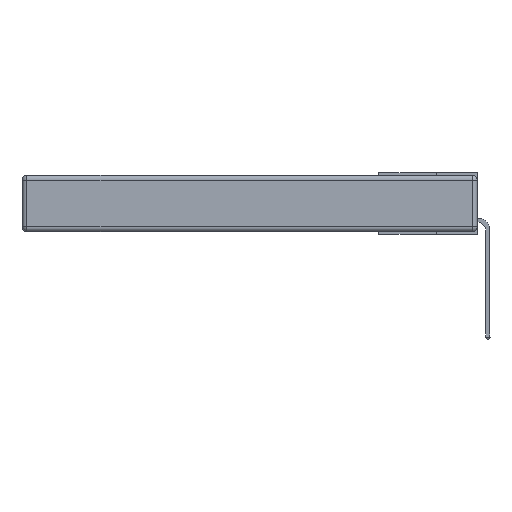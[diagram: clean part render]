
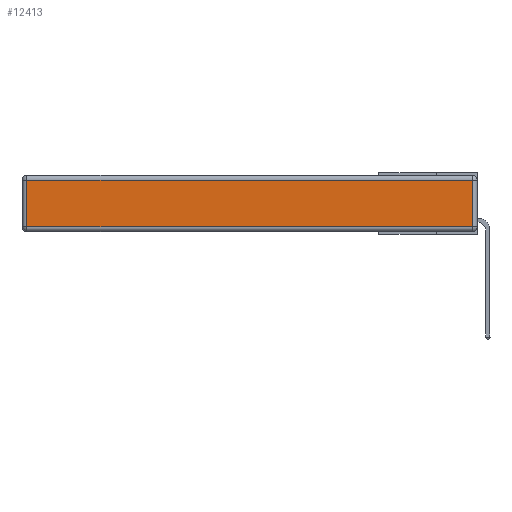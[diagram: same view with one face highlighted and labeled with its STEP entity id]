
A CAD part, left-side view. The second image highlights one B-rep face of the part: STEP entity #12413.
In plain terms, the highlighted planar face has unit normal (-1, 0, 0).
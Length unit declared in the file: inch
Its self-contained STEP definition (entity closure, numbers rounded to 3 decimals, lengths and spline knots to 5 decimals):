
#301 = CARTESIAN_POINT ( 'NONE',  ( 0., 2.75, -0.03 ) ) ;
#462 = LINE ( 'NONE', #27082, #18370 ) ;
#1208 = LINE ( 'NONE', #301, #10140 ) ;
#1718 = DIRECTION ( 'NONE',  ( -1., 0., 0. ) ) ;
#2941 = ORIENTED_EDGE ( 'NONE', *, *, #12968, .T. ) ;
#3369 = CARTESIAN_POINT ( 'NONE',  ( 0., 2.72, -0.03 ) ) ;
#3749 = VECTOR ( 'NONE', #17147, 39.37008 ) ;
#4694 = ORIENTED_EDGE ( 'NONE', *, *, #11218, .T. ) ;
#5098 = VERTEX_POINT ( 'NONE', #3369 ) ;
#5734 = CARTESIAN_POINT ( 'NONE',  ( 0., 0., -0.313 ) ) ;
#6032 = AXIS2_PLACEMENT_3D ( 'NONE', #13320, #1718, #24806 ) ;
#7993 = EDGE_CURVE ( 'NONE', #5098, #28779, #23115, .T. ) ;
#8801 = DIRECTION ( 'NONE',  ( 0., 0., -1. ) ) ;
#9459 = VERTEX_POINT ( 'NONE', #27248 ) ;
#10140 = VECTOR ( 'NONE', #11590, 39.37008 ) ;
#10469 = FACE_OUTER_BOUND ( 'NONE', #27353, .T. ) ;
#11218 = EDGE_CURVE ( 'NONE', #28779, #9459, #20643, .T. ) ;
#11470 = EDGE_CURVE ( 'NONE', #28701, #5098, #1208, .T. ) ;
#11590 = DIRECTION ( 'NONE',  ( 0., 1., 0. ) ) ;
#12413 = ADVANCED_FACE ( 'NONE', ( #10469 ), #15328, .T. ) ;
#12968 = EDGE_CURVE ( 'NONE', #9459, #28701, #462, .T. ) ;
#12983 = CARTESIAN_POINT ( 'NONE',  ( 0., 2.72, -0.313 ) ) ;
#13287 = DIRECTION ( 'NONE',  ( 0., 0., 1. ) ) ;
#13320 = CARTESIAN_POINT ( 'NONE',  ( 0., 0., -0.343 ) ) ;
#13616 = CARTESIAN_POINT ( 'NONE',  ( 0., 2.72, -0.343 ) ) ;
#15328 = PLANE ( 'NONE',  #6032 ) ;
#17147 = DIRECTION ( 'NONE',  ( 0., -1., 0. ) ) ;
#18370 = VECTOR ( 'NONE', #13287, 39.37008 ) ;
#20643 = LINE ( 'NONE', #5734, #3749 ) ;
#23115 = LINE ( 'NONE', #13616, #25245 ) ;
#24385 = CARTESIAN_POINT ( 'NONE',  ( 0., 0.03, -0.03 ) ) ;
#24806 = DIRECTION ( 'NONE',  ( 0., 0., 1. ) ) ;
#25245 = VECTOR ( 'NONE', #8801, 39.37008 ) ;
#26892 = ORIENTED_EDGE ( 'NONE', *, *, #11470, .T. ) ;
#27082 = CARTESIAN_POINT ( 'NONE',  ( 0., 0.03, -0.343 ) ) ;
#27248 = CARTESIAN_POINT ( 'NONE',  ( 0., 0.03, -0.313 ) ) ;
#27353 = EDGE_LOOP ( 'NONE', ( #4694, #2941, #26892, #29664 ) ) ;
#28701 = VERTEX_POINT ( 'NONE', #24385 ) ;
#28779 = VERTEX_POINT ( 'NONE', #12983 ) ;
#29664 = ORIENTED_EDGE ( 'NONE', *, *, #7993, .T. ) ;
